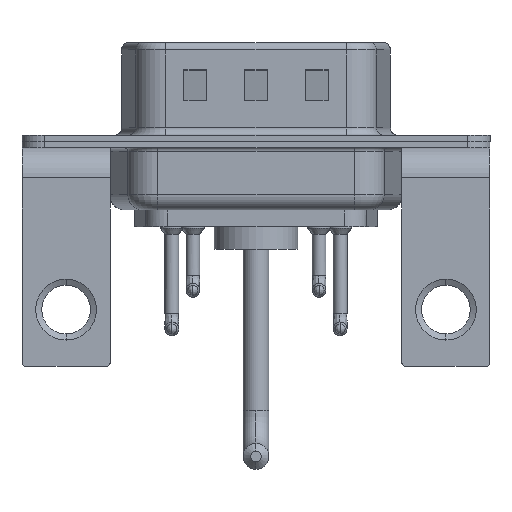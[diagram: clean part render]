
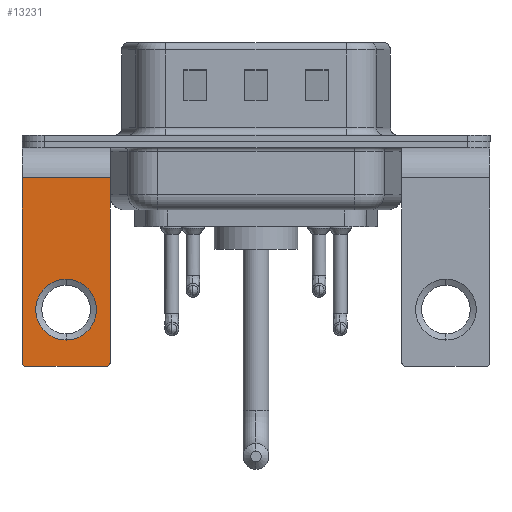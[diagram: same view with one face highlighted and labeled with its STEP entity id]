
A CAD part, front view. The second image highlights one B-rep face of the part: STEP entity #13231.
In plain terms, the highlighted planar face has unit normal (0, -1, 0).
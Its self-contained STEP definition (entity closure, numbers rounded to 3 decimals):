
#300 = ORIENTED_EDGE ( 'NONE', *, *, #7754, .T. ) ;
#841 = DIRECTION ( 'NONE',  ( 0., 0., -1. ) ) ;
#941 = VERTEX_POINT ( 'NONE', #19859 ) ;
#961 = LINE ( 'NONE', #16108, #12208 ) ;
#1847 = AXIS2_PLACEMENT_3D ( 'NONE', #7437, #15268, #18633 ) ;
#2152 = VECTOR ( 'NONE', #8988, 1000. ) ;
#2232 = DIRECTION ( 'NONE',  ( -1., 0., 0. ) ) ;
#2782 = LINE ( 'NONE', #20071, #2152 ) ;
#2841 = CARTESIAN_POINT ( 'NONE',  ( 0., -6.25, -11.07 ) ) ;
#3171 = ORIENTED_EDGE ( 'NONE', *, *, #5186, .T. ) ;
#3203 = DIRECTION ( 'NONE',  ( 0., 0., 1. ) ) ;
#3302 = CARTESIAN_POINT ( 'NONE',  ( 0., -6.25, -9.07 ) ) ;
#3758 = AXIS2_PLACEMENT_3D ( 'NONE', #13959, #6319, #16901 ) ;
#4015 = CARTESIAN_POINT ( 'NONE',  ( 2.9, -6.25, -2.4 ) ) ;
#4629 = DIRECTION ( 'NONE',  ( 0., 1., 0. ) ) ;
#4802 = VERTEX_POINT ( 'NONE', #3302 ) ;
#5068 = CARTESIAN_POINT ( 'NONE',  ( 0., -6.25, -11.07 ) ) ;
#5186 = EDGE_CURVE ( 'NONE', #12919, #12196, #9607, .T. ) ;
#5191 = AXIS2_PLACEMENT_3D ( 'NONE', #2841, #19717, #13630 ) ;
#5983 = EDGE_LOOP ( 'NONE', ( #300, #16148 ) ) ;
#6025 = CIRCLE ( 'NONE', #1847, 0.25 ) ;
#6185 = VERTEX_POINT ( 'NONE', #15218 ) ;
#6319 = DIRECTION ( 'NONE',  ( 0., -1., 0. ) ) ;
#6602 = DIRECTION ( 'NONE',  ( 0., 0., 1. ) ) ;
#7061 = VECTOR ( 'NONE', #2232, 1000. ) ;
#7123 = CIRCLE ( 'NONE', #5191, 2. ) ;
#7149 = LINE ( 'NONE', #4015, #12314 ) ;
#7437 = CARTESIAN_POINT ( 'NONE',  ( 2.65, -6.25, -14.55 ) ) ;
#7450 = EDGE_CURVE ( 'NONE', #941, #13120, #13319, .T. ) ;
#7677 = CARTESIAN_POINT ( 'NONE',  ( 2.9, -6.25, -2.4 ) ) ;
#7694 = ORIENTED_EDGE ( 'NONE', *, *, #8753, .F. ) ;
#7754 = EDGE_CURVE ( 'NONE', #6185, #4802, #11613, .T. ) ;
#7785 = FACE_BOUND ( 'NONE', #5983, .T. ) ;
#8753 = EDGE_CURVE ( 'NONE', #941, #9512, #7149, .T. ) ;
#8988 = DIRECTION ( 'NONE',  ( -1., 0., 0. ) ) ;
#9308 = FACE_OUTER_BOUND ( 'NONE', #11497, .T. ) ;
#9410 = EDGE_CURVE ( 'NONE', #4802, #6185, #7123, .T. ) ;
#9512 = VERTEX_POINT ( 'NONE', #14233 ) ;
#9607 = CIRCLE ( 'NONE', #3758, 0.25 ) ;
#10163 = CARTESIAN_POINT ( 'NONE',  ( 2.9, -6.25, -2.4 ) ) ;
#11074 = DIRECTION ( 'NONE',  ( 0., 1., 0. ) ) ;
#11242 = CARTESIAN_POINT ( 'NONE',  ( -2.9, -6.25, -14.55 ) ) ;
#11497 = EDGE_LOOP ( 'NONE', ( #11945, #3171, #14450, #19622, #7694, #17776 ) ) ;
#11613 = CIRCLE ( 'NONE', #17799, 2. ) ;
#11625 = DIRECTION ( 'NONE',  ( 0., 0., -1. ) ) ;
#11945 = ORIENTED_EDGE ( 'NONE', *, *, #18133, .T. ) ;
#11964 = CARTESIAN_POINT ( 'NONE',  ( 2.65, -6.25, -14.8 ) ) ;
#12196 = VERTEX_POINT ( 'NONE', #17822 ) ;
#12208 = VECTOR ( 'NONE', #11625, 1000. ) ;
#12314 = VECTOR ( 'NONE', #841, 1000. ) ;
#12919 = VERTEX_POINT ( 'NONE', #11242 ) ;
#13120 = VERTEX_POINT ( 'NONE', #19879 ) ;
#13231 = ADVANCED_FACE ( 'NONE', ( #7785, #9308 ), #17129, .F. ) ;
#13319 = LINE ( 'NONE', #10163, #7061 ) ;
#13347 = VERTEX_POINT ( 'NONE', #11964 ) ;
#13630 = DIRECTION ( 'NONE',  ( 0., 0., 1. ) ) ;
#13959 = CARTESIAN_POINT ( 'NONE',  ( -2.65, -6.25, -14.55 ) ) ;
#14233 = CARTESIAN_POINT ( 'NONE',  ( 2.9, -6.25, -14.55 ) ) ;
#14450 = ORIENTED_EDGE ( 'NONE', *, *, #18393, .F. ) ;
#15218 = CARTESIAN_POINT ( 'NONE',  ( 0., -6.25, -13.07 ) ) ;
#15268 = DIRECTION ( 'NONE',  ( 0., -1., 0. ) ) ;
#16108 = CARTESIAN_POINT ( 'NONE',  ( -2.9, -6.25, -2.4 ) ) ;
#16148 = ORIENTED_EDGE ( 'NONE', *, *, #9410, .T. ) ;
#16901 = DIRECTION ( 'NONE',  ( 0., 0., 1. ) ) ;
#17073 = EDGE_CURVE ( 'NONE', #13347, #9512, #6025, .T. ) ;
#17129 = PLANE ( 'NONE',  #17555 ) ;
#17555 = AXIS2_PLACEMENT_3D ( 'NONE', #7677, #4629, #3203 ) ;
#17776 = ORIENTED_EDGE ( 'NONE', *, *, #7450, .T. ) ;
#17799 = AXIS2_PLACEMENT_3D ( 'NONE', #5068, #11074, #6602 ) ;
#17822 = CARTESIAN_POINT ( 'NONE',  ( -2.65, -6.25, -14.8 ) ) ;
#18133 = EDGE_CURVE ( 'NONE', #13120, #12919, #961, .T. ) ;
#18393 = EDGE_CURVE ( 'NONE', #13347, #12196, #2782, .T. ) ;
#18633 = DIRECTION ( 'NONE',  ( 0., 0., 1. ) ) ;
#19622 = ORIENTED_EDGE ( 'NONE', *, *, #17073, .T. ) ;
#19717 = DIRECTION ( 'NONE',  ( 0., 1., 0. ) ) ;
#19859 = CARTESIAN_POINT ( 'NONE',  ( 2.9, -6.25, -2.4 ) ) ;
#19879 = CARTESIAN_POINT ( 'NONE',  ( -2.9, -6.25, -2.4 ) ) ;
#20071 = CARTESIAN_POINT ( 'NONE',  ( 2.9, -6.25, -14.8 ) ) ;
